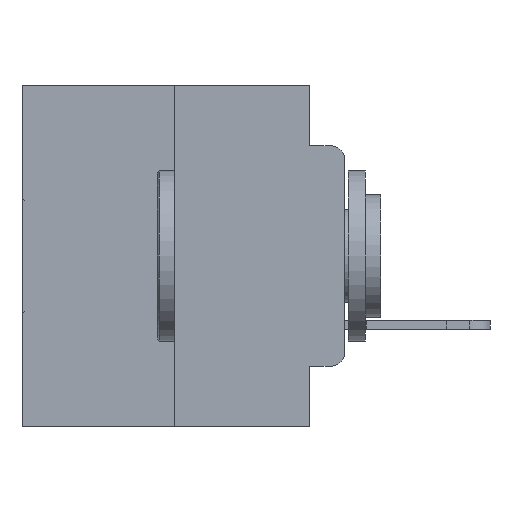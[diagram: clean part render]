
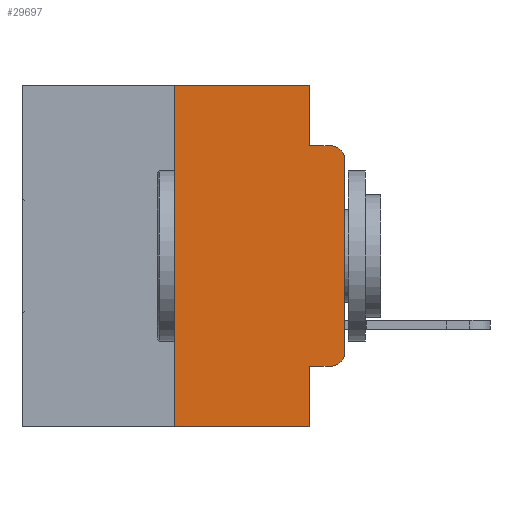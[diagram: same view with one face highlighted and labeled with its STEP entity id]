
A CAD part, left-side view. The second image highlights one B-rep face of the part: STEP entity #29697.
In plain terms, the highlighted planar face has unit normal (-1, 0, 0).
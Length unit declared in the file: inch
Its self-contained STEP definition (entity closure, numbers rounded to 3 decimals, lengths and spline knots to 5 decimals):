
#10 = VERTEX_POINT ( 'NONE', #171 ) ;
#45 = DIRECTION ( 'NONE',  ( 0., 0., 1. ) ) ;
#171 = CARTESIAN_POINT ( 'NONE',  ( 0., 0.02, -0.0885 ) ) ;
#423 = ORIENTED_EDGE ( 'NONE', *, *, #2665, .F. ) ;
#728 = VERTEX_POINT ( 'NONE', #13217 ) ;
#823 = ORIENTED_EDGE ( 'NONE', *, *, #28160, .F. ) ;
#1289 = CIRCLE ( 'NONE', #12798, 0.02 ) ;
#1652 = DIRECTION ( 'NONE',  ( 0., 0., -1. ) ) ;
#1728 = LINE ( 'NONE', #28306, #14004 ) ;
#2093 = DIRECTION ( 'NONE',  ( 0., 0., -1. ) ) ;
#2325 = VECTOR ( 'NONE', #12730, 39.37008 ) ;
#2376 = EDGE_CURVE ( 'NONE', #25069, #7650, #18272, .T. ) ;
#2665 = EDGE_CURVE ( 'NONE', #23720, #25069, #15655, .T. ) ;
#3408 = CARTESIAN_POINT ( 'NONE',  ( 0., 0.02, -0.1085 ) ) ;
#4742 = ORIENTED_EDGE ( 'NONE', *, *, #21375, .T. ) ;
#4956 = CARTESIAN_POINT ( 'NONE',  ( 0., 0.051, -0.0885 ) ) ;
#5144 = CARTESIAN_POINT ( 'NONE',  ( 0., 0.473, 0. ) ) ;
#5325 = AXIS2_PLACEMENT_3D ( 'NONE', #5144, #21771, #7589 ) ;
#5966 = DIRECTION ( 'NONE',  ( 0., 0., -1. ) ) ;
#6142 = CARTESIAN_POINT ( 'NONE',  ( 0., 0.051, -0.4115 ) ) ;
#6608 = VERTEX_POINT ( 'NONE', #27587 ) ;
#7278 = VERTEX_POINT ( 'NONE', #13420 ) ;
#7384 = EDGE_CURVE ( 'NONE', #7650, #10, #28440, .T. ) ;
#7589 = DIRECTION ( 'NONE',  ( 0., 0., -1. ) ) ;
#7606 = VERTEX_POINT ( 'NONE', #6142 ) ;
#7650 = VERTEX_POINT ( 'NONE', #4956 ) ;
#7986 = EDGE_CURVE ( 'NONE', #7606, #7278, #27319, .T. ) ;
#8173 = LINE ( 'NONE', #10352, #2325 ) ;
#8561 = VECTOR ( 'NONE', #28439, 39.37008 ) ;
#8631 = VERTEX_POINT ( 'NONE', #26333 ) ;
#9274 = CARTESIAN_POINT ( 'NONE',  ( 0., 0.25, 0. ) ) ;
#9369 = VECTOR ( 'NONE', #10840, 39.37008 ) ;
#9450 = ORIENTED_EDGE ( 'NONE', *, *, #22259, .F. ) ;
#10352 = CARTESIAN_POINT ( 'NONE',  ( 0., 0.473, -0.5 ) ) ;
#10840 = DIRECTION ( 'NONE',  ( 0., -1., 0. ) ) ;
#10915 = CARTESIAN_POINT ( 'NONE',  ( 0., 0.051, -0.0885 ) ) ;
#11974 = VECTOR ( 'NONE', #2093, 39.37008 ) ;
#12252 = EDGE_CURVE ( 'NONE', #23185, #10, #29436, .T. ) ;
#12730 = DIRECTION ( 'NONE',  ( 0., -1., 0. ) ) ;
#12798 = AXIS2_PLACEMENT_3D ( 'NONE', #29674, #16261, #1652 ) ;
#13217 = CARTESIAN_POINT ( 'NONE',  ( 0., 0., -0.3915 ) ) ;
#13420 = CARTESIAN_POINT ( 'NONE',  ( 0., 0.02, -0.4115 ) ) ;
#13616 = CARTESIAN_POINT ( 'NONE',  ( 0., 0.25, 0. ) ) ;
#14000 = CARTESIAN_POINT ( 'NONE',  ( 0., 0.051, 0. ) ) ;
#14004 = VECTOR ( 'NONE', #45, 39.37008 ) ;
#14935 = ORIENTED_EDGE ( 'NONE', *, *, #7986, .T. ) ;
#15387 = CARTESIAN_POINT ( 'NONE',  ( 0., 0.473, 0. ) ) ;
#15655 = LINE ( 'NONE', #15387, #8561 ) ;
#16257 = AXIS2_PLACEMENT_3D ( 'NONE', #3408, #20202, #5966 ) ;
#16261 = DIRECTION ( 'NONE',  ( -1., 0., 0. ) ) ;
#17009 = EDGE_CURVE ( 'NONE', #728, #23185, #1728, .T. ) ;
#17077 = LINE ( 'NONE', #13616, #22516 ) ;
#17589 = EDGE_LOOP ( 'NONE', ( #17991, #20893, #20603, #22161, #423, #823, #4742, #9450, #14935, #17844 ) ) ;
#17627 = CARTESIAN_POINT ( 'NONE',  ( 0., 0.051, 0. ) ) ;
#17844 = ORIENTED_EDGE ( 'NONE', *, *, #30055, .T. ) ;
#17991 = ORIENTED_EDGE ( 'NONE', *, *, #17009, .T. ) ;
#18272 = LINE ( 'NONE', #17627, #11974 ) ;
#19443 = PLANE ( 'NONE',  #5325 ) ;
#20202 = DIRECTION ( 'NONE',  ( -1., 0., 0. ) ) ;
#20520 = DIRECTION ( 'NONE',  ( 0., 0., -1. ) ) ;
#20603 = ORIENTED_EDGE ( 'NONE', *, *, #7384, .F. ) ;
#20893 = ORIENTED_EDGE ( 'NONE', *, *, #12252, .T. ) ;
#21264 = CARTESIAN_POINT ( 'NONE',  ( 0., 0., -0.1085 ) ) ;
#21328 = FACE_OUTER_BOUND ( 'NONE', #17589, .T. ) ;
#21375 = EDGE_CURVE ( 'NONE', #8631, #6608, #8173, .T. ) ;
#21431 = LINE ( 'NONE', #27156, #26656 ) ;
#21771 = DIRECTION ( 'NONE',  ( 1., 0., 0. ) ) ;
#22146 = VECTOR ( 'NONE', #26115, 39.37008 ) ;
#22161 = ORIENTED_EDGE ( 'NONE', *, *, #2376, .F. ) ;
#22259 = EDGE_CURVE ( 'NONE', #7606, #6608, #21431, .T. ) ;
#22516 = VECTOR ( 'NONE', #29447, 39.37008 ) ;
#23185 = VERTEX_POINT ( 'NONE', #21264 ) ;
#23720 = VERTEX_POINT ( 'NONE', #9274 ) ;
#25069 = VERTEX_POINT ( 'NONE', #14000 ) ;
#25951 = CARTESIAN_POINT ( 'NONE',  ( 0., 0.051, -0.4115 ) ) ;
#26115 = DIRECTION ( 'NONE',  ( 0., -1., 0. ) ) ;
#26333 = CARTESIAN_POINT ( 'NONE',  ( 0., 0.25, -0.5 ) ) ;
#26656 = VECTOR ( 'NONE', #20520, 39.37008 ) ;
#27156 = CARTESIAN_POINT ( 'NONE',  ( 0., 0.051, 0. ) ) ;
#27319 = LINE ( 'NONE', #25951, #22146 ) ;
#27587 = CARTESIAN_POINT ( 'NONE',  ( 0., 0.051, -0.5 ) ) ;
#28160 = EDGE_CURVE ( 'NONE', #8631, #23720, #17077, .T. ) ;
#28306 = CARTESIAN_POINT ( 'NONE',  ( 0., 0., 0. ) ) ;
#28439 = DIRECTION ( 'NONE',  ( 0., -1., 0. ) ) ;
#28440 = LINE ( 'NONE', #10915, #9369 ) ;
#29436 = CIRCLE ( 'NONE', #16257, 0.02 ) ;
#29447 = DIRECTION ( 'NONE',  ( 0., 0., 1. ) ) ;
#29674 = CARTESIAN_POINT ( 'NONE',  ( 0., 0.02, -0.3915 ) ) ;
#29697 = ADVANCED_FACE ( 'NONE', ( #21328 ), #19443, .F. ) ;
#30055 = EDGE_CURVE ( 'NONE', #7278, #728, #1289, .T. ) ;
